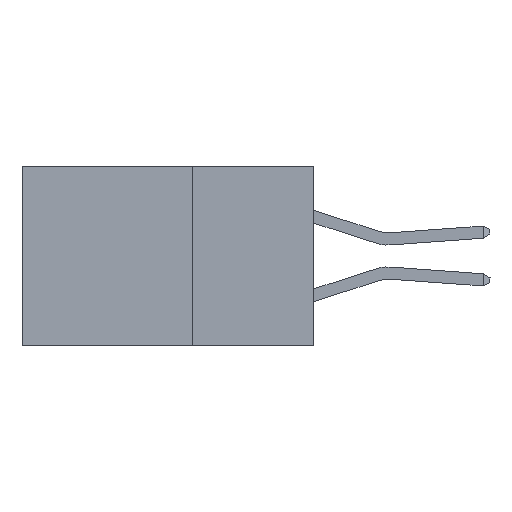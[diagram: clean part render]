
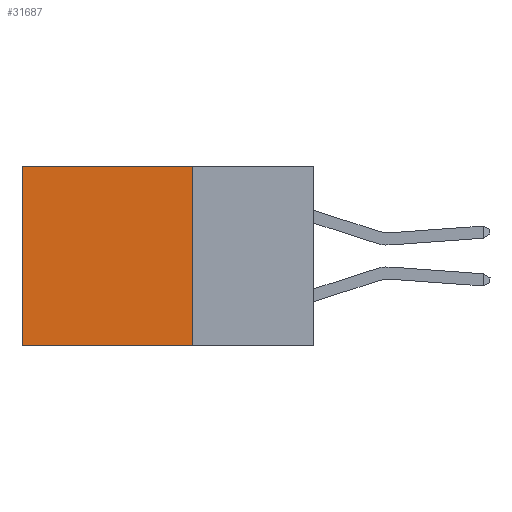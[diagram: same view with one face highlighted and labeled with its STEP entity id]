
A CAD part, left-side view. The second image highlights one B-rep face of the part: STEP entity #31687.
In plain terms, the highlighted planar face has unit normal (-1, 0, 0).
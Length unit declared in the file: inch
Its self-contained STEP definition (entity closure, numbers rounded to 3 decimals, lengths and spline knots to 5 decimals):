
#633 = CARTESIAN_POINT ( 'NONE',  ( 0.2875, 0.6, 0. ) ) ;
#1595 = VERTEX_POINT ( 'NONE', #25185 ) ;
#2595 = ORIENTED_EDGE ( 'NONE', *, *, #5370, .T. ) ;
#3082 = DIRECTION ( 'NONE',  ( 0., 0., -1. ) ) ;
#4876 = LINE ( 'NONE', #13766, #23241 ) ;
#5370 = EDGE_CURVE ( 'NONE', #1595, #14250, #4876, .T. ) ;
#8524 = LINE ( 'NONE', #633, #22939 ) ;
#9147 = VECTOR ( 'NONE', #21975, 39.37008 ) ;
#11961 = ORIENTED_EDGE ( 'NONE', *, *, #26536, .F. ) ;
#12690 = AXIS2_PLACEMENT_3D ( 'NONE', #16977, #16744, #3082 ) ;
#12755 = LINE ( 'NONE', #20515, #27155 ) ;
#13766 = CARTESIAN_POINT ( 'NONE',  ( 0.2875, 0.25, 0. ) ) ;
#14250 = VERTEX_POINT ( 'NONE', #34002 ) ;
#14495 = VERTEX_POINT ( 'NONE', #18193 ) ;
#14763 = DIRECTION ( 'NONE',  ( 0., 1., 0. ) ) ;
#15859 = ORIENTED_EDGE ( 'NONE', *, *, #35977, .F. ) ;
#16744 = DIRECTION ( 'NONE',  ( 1., 0., 0. ) ) ;
#16977 = CARTESIAN_POINT ( 'NONE',  ( 0.2875, 0.25, 0. ) ) ;
#17448 = VERTEX_POINT ( 'NONE', #31480 ) ;
#18193 = CARTESIAN_POINT ( 'NONE',  ( 0.2875, 0.6, -0.37 ) ) ;
#20515 = CARTESIAN_POINT ( 'NONE',  ( 0.2875, 0.25, -0.37 ) ) ;
#21975 = DIRECTION ( 'NONE',  ( 0., 0., -1. ) ) ;
#22939 = VECTOR ( 'NONE', #25793, 39.37008 ) ;
#23241 = VECTOR ( 'NONE', #27812, 39.37008 ) ;
#24557 = CARTESIAN_POINT ( 'NONE',  ( 0.2875, 0.25, 0. ) ) ;
#25185 = CARTESIAN_POINT ( 'NONE',  ( 0.2875, 0.25, 0. ) ) ;
#25793 = DIRECTION ( 'NONE',  ( 0., 0., -1. ) ) ;
#26536 = EDGE_CURVE ( 'NONE', #17448, #14495, #12755, .T. ) ;
#27030 = ORIENTED_EDGE ( 'NONE', *, *, #31779, .T. ) ;
#27155 = VECTOR ( 'NONE', #14763, 39.37008 ) ;
#27812 = DIRECTION ( 'NONE',  ( 0., 1., 0. ) ) ;
#27873 = LINE ( 'NONE', #24557, #9147 ) ;
#29941 = EDGE_LOOP ( 'NONE', ( #27030, #11961, #15859, #2595 ) ) ;
#30809 = FACE_OUTER_BOUND ( 'NONE', #29941, .T. ) ;
#31480 = CARTESIAN_POINT ( 'NONE',  ( 0.2875, 0.25, -0.37 ) ) ;
#31687 = ADVANCED_FACE ( 'NONE', ( #30809 ), #33763, .F. ) ;
#31779 = EDGE_CURVE ( 'NONE', #14250, #14495, #8524, .T. ) ;
#33763 = PLANE ( 'NONE',  #12690 ) ;
#34002 = CARTESIAN_POINT ( 'NONE',  ( 0.2875, 0.6, 0. ) ) ;
#35977 = EDGE_CURVE ( 'NONE', #1595, #17448, #27873, .T. ) ;
